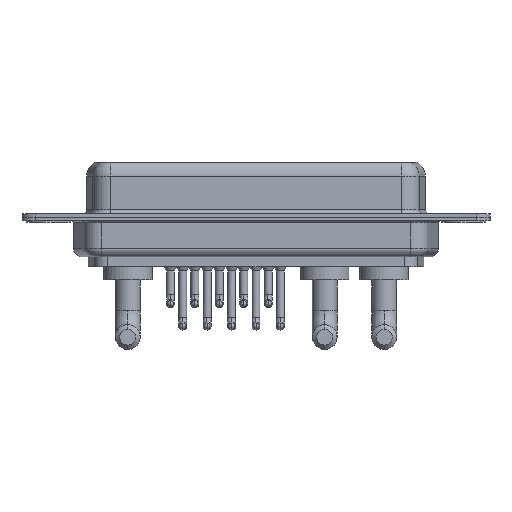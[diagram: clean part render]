
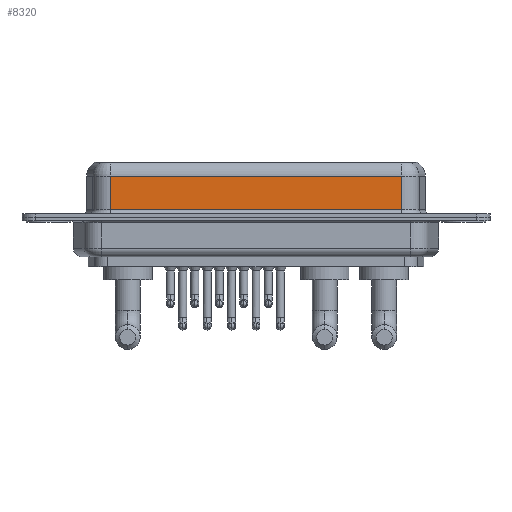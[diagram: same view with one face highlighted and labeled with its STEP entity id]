
A CAD part, front view. The second image highlights one B-rep face of the part: STEP entity #8320.
In plain terms, the highlighted planar face has unit normal (0, -1, 0).
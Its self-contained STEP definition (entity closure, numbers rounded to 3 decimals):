
#854 = CARTESIAN_POINT ( 'NONE',  ( 7.013, -3.95, 6.4 ) ) ;
#883 = CARTESIAN_POINT ( 'NONE',  ( 40.037, -3.95, 0.9 ) ) ;
#1391 = DIRECTION ( 'NONE',  ( 0., 0., -1. ) ) ;
#2192 = ORIENTED_EDGE ( 'NONE', *, *, #14782, .T. ) ;
#2297 = DIRECTION ( 'NONE',  ( 0., 0., 1. ) ) ;
#2405 = CARTESIAN_POINT ( 'NONE',  ( 40.037, -3.95, 4.65 ) ) ;
#2472 = PLANE ( 'NONE',  #8056 ) ;
#2529 = LINE ( 'NONE', #5240, #13784 ) ;
#2611 = DIRECTION ( 'NONE',  ( 1., 0., 0. ) ) ;
#2943 = VECTOR ( 'NONE', #14909, 1000. ) ;
#3828 = EDGE_CURVE ( 'NONE', #17228, #8310, #8039, .T. ) ;
#4010 = VECTOR ( 'NONE', #8470, 1000. ) ;
#4116 = ORIENTED_EDGE ( 'NONE', *, *, #14044, .T. ) ;
#5240 = CARTESIAN_POINT ( 'NONE',  ( 40.037, -3.95, 0.9 ) ) ;
#5431 = CARTESIAN_POINT ( 'NONE',  ( 40.037, -3.95, 6.4 ) ) ;
#6364 = VERTEX_POINT ( 'NONE', #10810 ) ;
#6872 = EDGE_LOOP ( 'NONE', ( #10648, #15290, #2192, #4116 ) ) ;
#8039 = LINE ( 'NONE', #5431, #15622 ) ;
#8056 = AXIS2_PLACEMENT_3D ( 'NONE', #14265, #12693, #2297 ) ;
#8310 = VERTEX_POINT ( 'NONE', #883 ) ;
#8320 = ADVANCED_FACE ( 'NONE', ( #14436 ), #2472, .F. ) ;
#8470 = DIRECTION ( 'NONE',  ( 0., 0., -1. ) ) ;
#9663 = LINE ( 'NONE', #13596, #2943 ) ;
#10130 = LINE ( 'NONE', #854, #4010 ) ;
#10214 = VERTEX_POINT ( 'NONE', #13709 ) ;
#10648 = ORIENTED_EDGE ( 'NONE', *, *, #3828, .F. ) ;
#10810 = CARTESIAN_POINT ( 'NONE',  ( 7.013, -3.95, 4.65 ) ) ;
#12693 = DIRECTION ( 'NONE',  ( 0., 1., 0. ) ) ;
#13596 = CARTESIAN_POINT ( 'NONE',  ( 40.037, -3.95, 4.65 ) ) ;
#13709 = CARTESIAN_POINT ( 'NONE',  ( 7.013, -3.95, 0.9 ) ) ;
#13784 = VECTOR ( 'NONE', #2611, 1000. ) ;
#14044 = EDGE_CURVE ( 'NONE', #10214, #8310, #2529, .T. ) ;
#14265 = CARTESIAN_POINT ( 'NONE',  ( 40.037, -3.95, 6.4 ) ) ;
#14436 = FACE_OUTER_BOUND ( 'NONE', #6872, .T. ) ;
#14782 = EDGE_CURVE ( 'NONE', #6364, #10214, #10130, .T. ) ;
#14909 = DIRECTION ( 'NONE',  ( -1., 0., 0. ) ) ;
#15290 = ORIENTED_EDGE ( 'NONE', *, *, #16798, .T. ) ;
#15622 = VECTOR ( 'NONE', #1391, 1000. ) ;
#16798 = EDGE_CURVE ( 'NONE', #17228, #6364, #9663, .T. ) ;
#17228 = VERTEX_POINT ( 'NONE', #2405 ) ;
